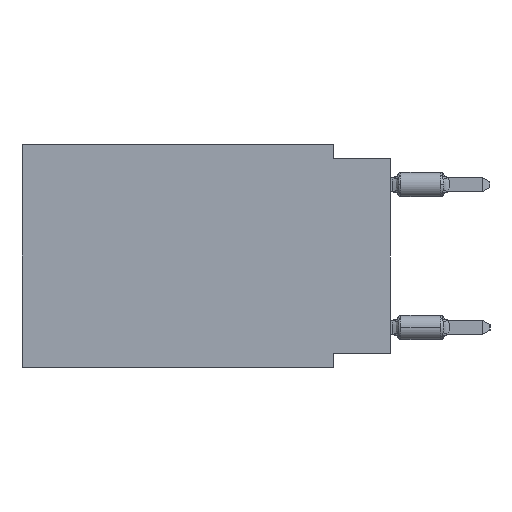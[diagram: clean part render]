
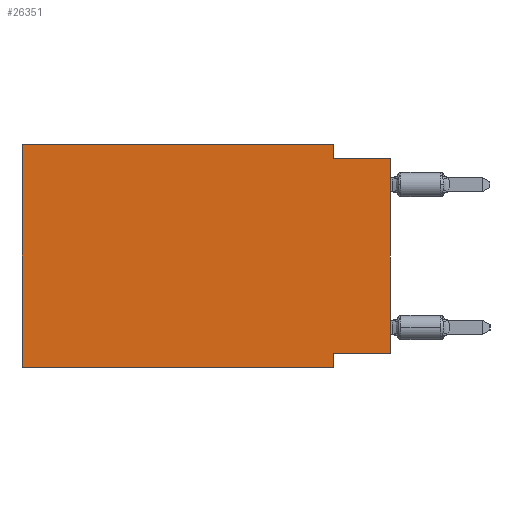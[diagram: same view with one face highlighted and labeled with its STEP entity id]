
A CAD part, left-side view. The second image highlights one B-rep face of the part: STEP entity #26351.
In plain terms, the highlighted planar face has unit normal (-1, 0, 0).
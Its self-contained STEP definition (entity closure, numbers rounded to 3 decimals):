
#335 = VECTOR ( 'NONE', #11975, 1000. ) ;
#487 = DIRECTION ( 'NONE',  ( 1., 0., 0. ) ) ;
#1016 = EDGE_CURVE ( 'NONE', #23748, #15499, #37953, .T. ) ;
#1602 = CARTESIAN_POINT ( 'NONE',  ( 0., 0., -0.635 ) ) ;
#2243 = VECTOR ( 'NONE', #5630, 1000. ) ;
#2378 = CARTESIAN_POINT ( 'NONE',  ( 0., 2.54, -9.906 ) ) ;
#2865 = CARTESIAN_POINT ( 'NONE',  ( 0., 2.54, -9.906 ) ) ;
#3030 = FACE_OUTER_BOUND ( 'NONE', #34861, .T. ) ;
#3262 = EDGE_CURVE ( 'NONE', #10952, #30542, #29888, .T. ) ;
#3484 = DIRECTION ( 'NONE',  ( 0., 0., -1. ) ) ;
#5522 = CARTESIAN_POINT ( 'NONE',  ( 0., 16.383, 0. ) ) ;
#5592 = VECTOR ( 'NONE', #19204, 1000. ) ;
#5630 = DIRECTION ( 'NONE',  ( 0., -1., 0. ) ) ;
#5836 = VECTOR ( 'NONE', #38611, 1000. ) ;
#5903 = LINE ( 'NONE', #6107, #5592 ) ;
#6107 = CARTESIAN_POINT ( 'NONE',  ( 0., 0., 0. ) ) ;
#6718 = CARTESIAN_POINT ( 'NONE',  ( 0., 2.54, 0. ) ) ;
#7925 = LINE ( 'NONE', #24660, #335 ) ;
#8461 = VERTEX_POINT ( 'NONE', #2865 ) ;
#10120 = PLANE ( 'NONE',  #17513 ) ;
#10934 = EDGE_CURVE ( 'NONE', #29268, #8461, #31768, .T. ) ;
#10952 = VERTEX_POINT ( 'NONE', #21711 ) ;
#11975 = DIRECTION ( 'NONE',  ( 0., -1., 0. ) ) ;
#12109 = ORIENTED_EDGE ( 'NONE', *, *, #29385, .F. ) ;
#13273 = ORIENTED_EDGE ( 'NONE', *, *, #41099, .T. ) ;
#13550 = CARTESIAN_POINT ( 'NONE',  ( 0., 2.54, -0.635 ) ) ;
#13567 = CARTESIAN_POINT ( 'NONE',  ( 0., 0., -9.271 ) ) ;
#15499 = VERTEX_POINT ( 'NONE', #5522 ) ;
#15892 = VERTEX_POINT ( 'NONE', #31407 ) ;
#17376 = ORIENTED_EDGE ( 'NONE', *, *, #10934, .F. ) ;
#17513 = AXIS2_PLACEMENT_3D ( 'NONE', #23013, #487, #23421 ) ;
#17625 = VECTOR ( 'NONE', #34130, 1000. ) ;
#18319 = CARTESIAN_POINT ( 'NONE',  ( 0., 16.383, -9.906 ) ) ;
#19165 = ORIENTED_EDGE ( 'NONE', *, *, #36604, .F. ) ;
#19204 = DIRECTION ( 'NONE',  ( 0., 0., 1. ) ) ;
#19791 = LINE ( 'NONE', #13567, #22746 ) ;
#21711 = CARTESIAN_POINT ( 'NONE',  ( 0., 2.54, 0. ) ) ;
#21762 = LINE ( 'NONE', #1602, #2243 ) ;
#22164 = CARTESIAN_POINT ( 'NONE',  ( 0., 0., -0.635 ) ) ;
#22746 = VECTOR ( 'NONE', #30506, 1000. ) ;
#22945 = ORIENTED_EDGE ( 'NONE', *, *, #36357, .T. ) ;
#23013 = CARTESIAN_POINT ( 'NONE',  ( 0., 16.383, 0. ) ) ;
#23258 = ORIENTED_EDGE ( 'NONE', *, *, #35605, .F. ) ;
#23421 = DIRECTION ( 'NONE',  ( 0., 0., -1. ) ) ;
#23748 = VERTEX_POINT ( 'NONE', #18319 ) ;
#24660 = CARTESIAN_POINT ( 'NONE',  ( 0., 16.383, -9.906 ) ) ;
#26351 = ADVANCED_FACE ( 'NONE', ( #3030 ), #10120, .F. ) ;
#29224 = VECTOR ( 'NONE', #40979, 1000. ) ;
#29268 = VERTEX_POINT ( 'NONE', #29846 ) ;
#29385 = EDGE_CURVE ( 'NONE', #15499, #10952, #31329, .T. ) ;
#29846 = CARTESIAN_POINT ( 'NONE',  ( 0., 2.54, -9.271 ) ) ;
#29888 = LINE ( 'NONE', #6718, #31667 ) ;
#30506 = DIRECTION ( 'NONE',  ( 0., 1., 0. ) ) ;
#30542 = VERTEX_POINT ( 'NONE', #13550 ) ;
#31329 = LINE ( 'NONE', #31519, #17625 ) ;
#31407 = CARTESIAN_POINT ( 'NONE',  ( 0., 0., -9.271 ) ) ;
#31519 = CARTESIAN_POINT ( 'NONE',  ( 0., 16.383, 0. ) ) ;
#31667 = VECTOR ( 'NONE', #3484, 1000. ) ;
#31768 = LINE ( 'NONE', #2378, #5836 ) ;
#34130 = DIRECTION ( 'NONE',  ( 0., -1., 0. ) ) ;
#34541 = CARTESIAN_POINT ( 'NONE',  ( 0., 16.383, 0. ) ) ;
#34861 = EDGE_LOOP ( 'NONE', ( #22945, #19165, #39747, #12109, #41089, #13273, #17376, #23258 ) ) ;
#35605 = EDGE_CURVE ( 'NONE', #15892, #29268, #19791, .T. ) ;
#36357 = EDGE_CURVE ( 'NONE', #15892, #42069, #5903, .T. ) ;
#36604 = EDGE_CURVE ( 'NONE', #30542, #42069, #21762, .T. ) ;
#37953 = LINE ( 'NONE', #34541, #29224 ) ;
#38611 = DIRECTION ( 'NONE',  ( 0., 0., -1. ) ) ;
#39747 = ORIENTED_EDGE ( 'NONE', *, *, #3262, .F. ) ;
#40979 = DIRECTION ( 'NONE',  ( 0., 0., 1. ) ) ;
#41089 = ORIENTED_EDGE ( 'NONE', *, *, #1016, .F. ) ;
#41099 = EDGE_CURVE ( 'NONE', #23748, #8461, #7925, .T. ) ;
#42069 = VERTEX_POINT ( 'NONE', #22164 ) ;
